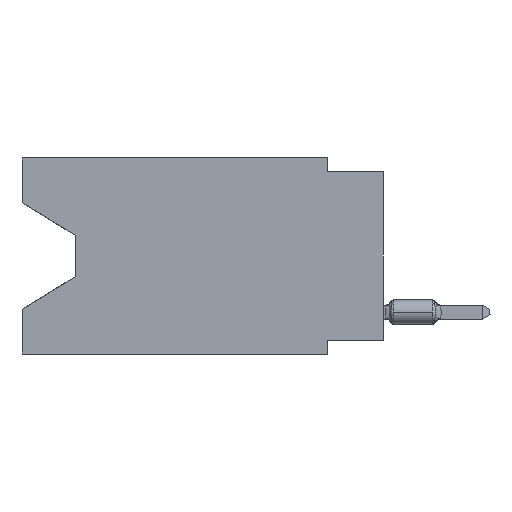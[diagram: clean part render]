
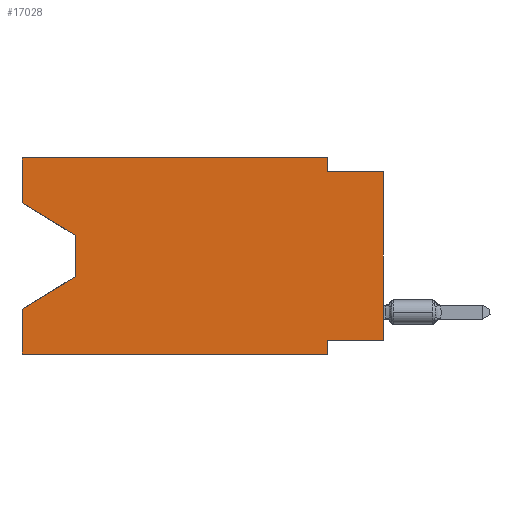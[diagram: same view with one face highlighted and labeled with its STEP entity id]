
A CAD part, left-side view. The second image highlights one B-rep face of the part: STEP entity #17028.
In plain terms, the highlighted planar face has unit normal (-1, 0, 0).
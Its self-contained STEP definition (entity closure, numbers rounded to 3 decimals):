
#106 = VECTOR ( 'NONE', #442, 1000. ) ;
#442 = DIRECTION ( 'NONE',  ( 0., 0., 1. ) ) ;
#1072 = CARTESIAN_POINT ( 'NONE',  ( 0., 0., -0.635 ) ) ;
#1086 = DIRECTION ( 'NONE',  ( 0., 0., -1. ) ) ;
#1415 = DIRECTION ( 'NONE',  ( 1., 0., 0. ) ) ;
#1593 = FACE_OUTER_BOUND ( 'NONE', #6292, .T. ) ;
#1606 = ORIENTED_EDGE ( 'NONE', *, *, #16520, .F. ) ;
#1608 = CARTESIAN_POINT ( 'NONE',  ( 0., 13.97, -3.505 ) ) ;
#1615 = ORIENTED_EDGE ( 'NONE', *, *, #19321, .F. ) ;
#2104 = ORIENTED_EDGE ( 'NONE', *, *, #16326, .T. ) ;
#2134 = ORIENTED_EDGE ( 'NONE', *, *, #23742, .F. ) ;
#2153 = DIRECTION ( 'NONE',  ( 0., 0., -1. ) ) ;
#3057 = LINE ( 'NONE', #21233, #106 ) ;
#3086 = VECTOR ( 'NONE', #29393, 1000. ) ;
#3502 = VERTEX_POINT ( 'NONE', #21072 ) ;
#3852 = DIRECTION ( 'NONE',  ( 0., 1., 0. ) ) ;
#4482 = LINE ( 'NONE', #31208, #22998 ) ;
#6292 = EDGE_LOOP ( 'NONE', ( #32472, #25879, #29849, #1615, #33585, #31843, #2134, #2104, #14888, #1606, #32274, #23777 ) ) ;
#6328 = VERTEX_POINT ( 'NONE', #9256 ) ;
#6366 = LINE ( 'NONE', #17036, #8682 ) ;
#6758 = DIRECTION ( 'NONE',  ( 0., 0.855, -0.519 ) ) ;
#6798 = DIRECTION ( 'NONE',  ( 0., 0., -1. ) ) ;
#7002 = PLANE ( 'NONE',  #13046 ) ;
#7011 = EDGE_CURVE ( 'NONE', #19543, #8265, #17458, .T. ) ;
#7729 = VECTOR ( 'NONE', #8946, 1000. ) ;
#8078 = CARTESIAN_POINT ( 'NONE',  ( 0., 16.383, -2.038 ) ) ;
#8265 = VERTEX_POINT ( 'NONE', #23632 ) ;
#8353 = CARTESIAN_POINT ( 'NONE',  ( 0., 16.383, -8.89 ) ) ;
#8682 = VECTOR ( 'NONE', #25069, 1000. ) ;
#8946 = DIRECTION ( 'NONE',  ( 0., -1., 0. ) ) ;
#9256 = CARTESIAN_POINT ( 'NONE',  ( 0., 16.383, 0. ) ) ;
#9590 = CARTESIAN_POINT ( 'NONE',  ( 0., 16.383, -8.89 ) ) ;
#11058 = CARTESIAN_POINT ( 'NONE',  ( 0., 13.97, -3.505 ) ) ;
#11891 = CARTESIAN_POINT ( 'NONE',  ( 0., 0., -0.635 ) ) ;
#13046 = AXIS2_PLACEMENT_3D ( 'NONE', #25349, #1415, #17666 ) ;
#14888 = ORIENTED_EDGE ( 'NONE', *, *, #33198, .F. ) ;
#15595 = VERTEX_POINT ( 'NONE', #29133 ) ;
#16326 = EDGE_CURVE ( 'NONE', #3502, #33994, #3057, .T. ) ;
#16461 = LINE ( 'NONE', #27124, #28003 ) ;
#16520 = EDGE_CURVE ( 'NONE', #31044, #15595, #20828, .T. ) ;
#17028 = ADVANCED_FACE ( 'NONE', ( #1593 ), #7002, .F. ) ;
#17036 = CARTESIAN_POINT ( 'NONE',  ( 0., 16.383, 0. ) ) ;
#17458 = LINE ( 'NONE', #32675, #21588 ) ;
#17638 = LINE ( 'NONE', #22364, #32847 ) ;
#17666 = DIRECTION ( 'NONE',  ( 0., 0., -1. ) ) ;
#17790 = DIRECTION ( 'NONE',  ( 0., -1., 0. ) ) ;
#19321 = EDGE_CURVE ( 'NONE', #27105, #33155, #6366, .T. ) ;
#19433 = DIRECTION ( 'NONE',  ( 0., 0., 1. ) ) ;
#19543 = VERTEX_POINT ( 'NONE', #29063 ) ;
#20497 = CARTESIAN_POINT ( 'NONE',  ( 0., 2.54, 0. ) ) ;
#20720 = LINE ( 'NONE', #31381, #21627 ) ;
#20828 = LINE ( 'NONE', #20497, #31058 ) ;
#21072 = CARTESIAN_POINT ( 'NONE',  ( 0., 0., -8.255 ) ) ;
#21233 = CARTESIAN_POINT ( 'NONE',  ( 0., 0., 0. ) ) ;
#21421 = EDGE_CURVE ( 'NONE', #27105, #8265, #33524, .T. ) ;
#21588 = VECTOR ( 'NONE', #6798, 1000. ) ;
#21627 = VECTOR ( 'NONE', #6758, 1000. ) ;
#22227 = LINE ( 'NONE', #11058, #25256 ) ;
#22364 = CARTESIAN_POINT ( 'NONE',  ( 0., 0., -8.255 ) ) ;
#22535 = EDGE_CURVE ( 'NONE', #25671, #33155, #20720, .T. ) ;
#22863 = CARTESIAN_POINT ( 'NONE',  ( 0., 2.54, 0. ) ) ;
#22998 = VECTOR ( 'NONE', #28577, 1000. ) ;
#23347 = VERTEX_POINT ( 'NONE', #1608 ) ;
#23632 = CARTESIAN_POINT ( 'NONE',  ( 0., 2.54, -8.89 ) ) ;
#23742 = EDGE_CURVE ( 'NONE', #3502, #19543, #17638, .T. ) ;
#23777 = ORIENTED_EDGE ( 'NONE', *, *, #30479, .F. ) ;
#24147 = CARTESIAN_POINT ( 'NONE',  ( 0., 16.383, -2.038 ) ) ;
#25006 = LINE ( 'NONE', #1072, #7729 ) ;
#25069 = DIRECTION ( 'NONE',  ( 0., 0., 1. ) ) ;
#25256 = VECTOR ( 'NONE', #1086, 1000. ) ;
#25349 = CARTESIAN_POINT ( 'NONE',  ( 0., 16.383, 0. ) ) ;
#25671 = VERTEX_POINT ( 'NONE', #34453 ) ;
#25879 = ORIENTED_EDGE ( 'NONE', *, *, #31571, .T. ) ;
#26834 = EDGE_CURVE ( 'NONE', #33029, #23347, #32017, .T. ) ;
#27105 = VERTEX_POINT ( 'NONE', #8353 ) ;
#27124 = CARTESIAN_POINT ( 'NONE',  ( 0., 16.383, 0. ) ) ;
#28003 = VECTOR ( 'NONE', #19433, 1000. ) ;
#28241 = VECTOR ( 'NONE', #17790, 1000. ) ;
#28577 = DIRECTION ( 'NONE',  ( 0., -1., 0. ) ) ;
#29063 = CARTESIAN_POINT ( 'NONE',  ( 0., 2.54, -8.255 ) ) ;
#29133 = CARTESIAN_POINT ( 'NONE',  ( 0., 2.54, -0.635 ) ) ;
#29393 = DIRECTION ( 'NONE',  ( 0., -0.855, -0.519 ) ) ;
#29849 = ORIENTED_EDGE ( 'NONE', *, *, #22535, .T. ) ;
#30479 = EDGE_CURVE ( 'NONE', #33029, #6328, #16461, .T. ) ;
#31044 = VERTEX_POINT ( 'NONE', #22863 ) ;
#31058 = VECTOR ( 'NONE', #2153, 1000. ) ;
#31208 = CARTESIAN_POINT ( 'NONE',  ( 0., 16.383, 0. ) ) ;
#31381 = CARTESIAN_POINT ( 'NONE',  ( 0., 13.97, -5.385 ) ) ;
#31571 = EDGE_CURVE ( 'NONE', #23347, #25671, #22227, .T. ) ;
#31843 = ORIENTED_EDGE ( 'NONE', *, *, #7011, .F. ) ;
#32017 = LINE ( 'NONE', #8078, #3086 ) ;
#32274 = ORIENTED_EDGE ( 'NONE', *, *, #32638, .F. ) ;
#32472 = ORIENTED_EDGE ( 'NONE', *, *, #26834, .T. ) ;
#32638 = EDGE_CURVE ( 'NONE', #6328, #31044, #4482, .T. ) ;
#32675 = CARTESIAN_POINT ( 'NONE',  ( 0., 2.54, -8.89 ) ) ;
#32847 = VECTOR ( 'NONE', #3852, 1000. ) ;
#33029 = VERTEX_POINT ( 'NONE', #24147 ) ;
#33155 = VERTEX_POINT ( 'NONE', #33557 ) ;
#33198 = EDGE_CURVE ( 'NONE', #15595, #33994, #25006, .T. ) ;
#33524 = LINE ( 'NONE', #9590, #28241 ) ;
#33557 = CARTESIAN_POINT ( 'NONE',  ( 0., 16.383, -6.852 ) ) ;
#33585 = ORIENTED_EDGE ( 'NONE', *, *, #21421, .T. ) ;
#33994 = VERTEX_POINT ( 'NONE', #11891 ) ;
#34453 = CARTESIAN_POINT ( 'NONE',  ( 0., 13.97, -5.385 ) ) ;
